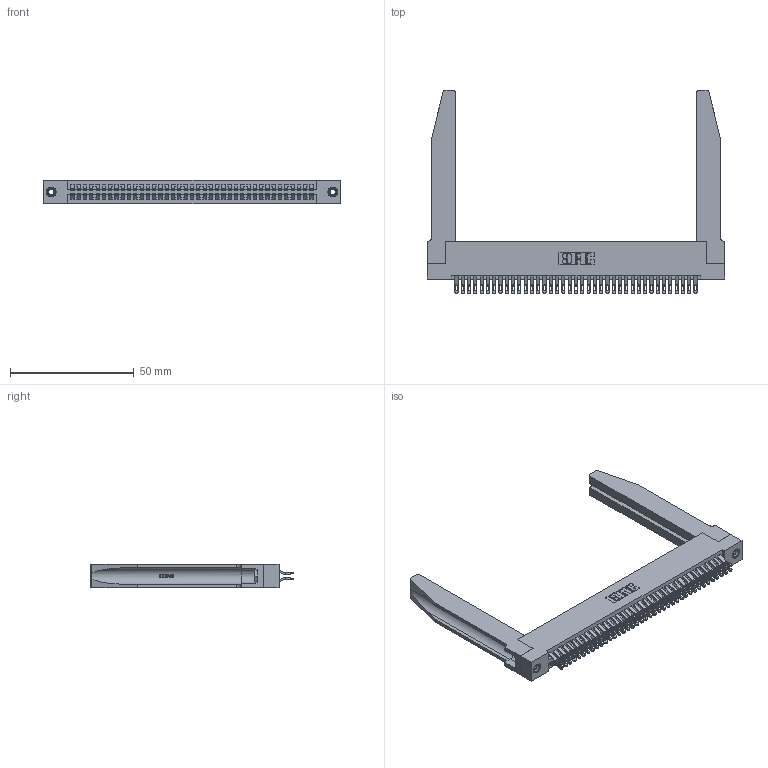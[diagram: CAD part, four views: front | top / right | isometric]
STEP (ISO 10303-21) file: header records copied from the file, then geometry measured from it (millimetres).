
FILE_DESCRIPTION (( 'STEP AP203' ), '1' );
FILE_NAME ('395-078-555-278.STEP', '2019-10-25T02:52:17', ( '' ), ( '' ), 'SwSTEP 2.0', 'SolidWorks 2016', '' );
FILE_SCHEMA (( 'CONFIG_CONTROL_DESIGN' ));
Length unit declared in the file: inch
Products named in the file (5): 345 Part_Flush Mounting Lugs - 0.156 Dia-TH; 345-292-001_555 Tail; 345-250-001_345-250-001-102; 345-220-078_345-220-078; 395-078-555-278
Assembly tree (83 placements, depth 2):
  395-078-555-278
    345 Part_Flush Mounting Lugs - 0.156 Dia-TH
    345-292-001_555 Tail  x78
    345-250-001_345-250-001-102  x2
    345-220-078_345-220-078  x2
Bounding box: 120.29 x 82.09 x 9.4 mm (x, y, z)
Volume: 19654.3 mm3; surface area: 25133.7 mm2
Topology: 83 solids, 83 shells, 4728 faces, 14755 edges, 9826 vertices
Faces by surface type: plane 2640, cylinder 2036, bspline 36, cone 12, torus 4
Entity records: 36070 total; most frequent: CARTESIAN_POINT 7001, ORIENTED_EDGE 5802, DIRECTION 5139, EDGE_CURVE 2901, LINE 2499, VECTOR 2499, VERTEX_POINT 1928, AXIS2_PLACEMENT_3D 1320
